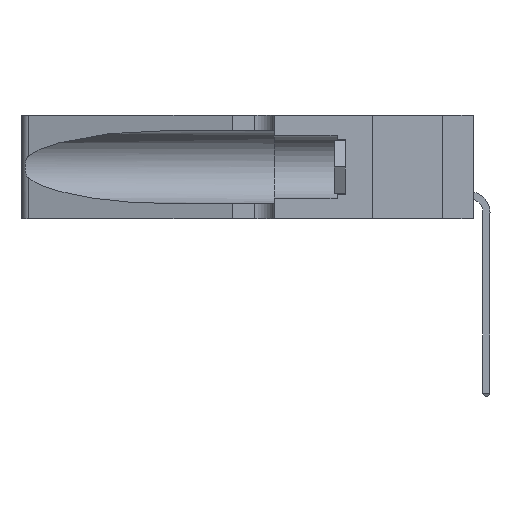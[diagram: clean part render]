
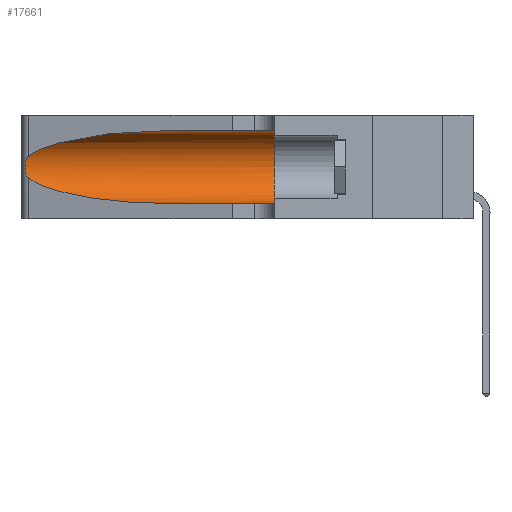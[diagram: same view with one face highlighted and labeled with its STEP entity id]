
A CAD part, left-side view. The second image highlights one B-rep face of the part: STEP entity #17661.
In plain terms, the highlighted cylindrical face has radius 3.308 mm (diameter 6.617 mm), a partial arc.
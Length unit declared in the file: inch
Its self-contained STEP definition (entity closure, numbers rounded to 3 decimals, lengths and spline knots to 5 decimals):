
#1006 = EDGE_CURVE ( 'NONE', #14968, #12927, #1416, .T. ) ;
#1194 = CARTESIAN_POINT ( 'NONE',  ( 0.25487, 1.22718, 0.14631 ) ) ;
#1416 =( BOUNDED_CURVE ( )  B_SPLINE_CURVE ( 3, ( #9014, #8951, #8760, #14597 ),
 .UNSPECIFIED., .F., .F. ) 
 B_SPLINE_CURVE_WITH_KNOTS ( ( 4, 4 ),
 ( 1.5708, 2.84003 ),
 .UNSPECIFIED. ) 
 CURVE ( )  GEOMETRIC_REPRESENTATION_ITEM ( )  RATIONAL_B_SPLINE_CURVE ( ( 1., 0.87, 0.87, 1. ) ) 
 REPRESENTATION_ITEM ( '' )  );
#1436 = EDGE_CURVE ( 'NONE', #14968, #13682, #16048, .T. ) ;
#2096 = CARTESIAN_POINT ( 'NONE',  ( 0.25639, 1.23186, 0.15144 ) ) ;
#2148 = CARTESIAN_POINT ( 'NONE',  ( 0.26017, 1.23833, 0.17102 ) ) ;
#2237 = VERTEX_POINT ( 'NONE', #12793 ) ;
#2344 = EDGE_LOOP ( 'NONE', ( #17675, #3521, #2361, #17129, #5200, #3640 ) ) ;
#2361 = ORIENTED_EDGE ( 'NONE', *, *, #11116, .T. ) ;
#2405 = DIRECTION ( 'NONE',  ( 0., -1., 0. ) ) ;
#2644 = CARTESIAN_POINT ( 'NONE',  ( 0.2373, 1.15595, 0.08982 ) ) ;
#3521 = ORIENTED_EDGE ( 'NONE', *, *, #12593, .T. ) ;
#3640 = ORIENTED_EDGE ( 'NONE', *, *, #1436, .F. ) ;
#4028 = DIRECTION ( 'NONE',  ( 0., 0., 1. ) ) ;
#4147 = DIRECTION ( 'NONE',  ( 0., 1., 0. ) ) ;
#5179 = CARTESIAN_POINT ( 'NONE',  ( 0.1305, 1.61858, 0.185 ) ) ;
#5200 = ORIENTED_EDGE ( 'NONE', *, *, #14529, .F. ) ;
#5296 =( BOUNDED_CURVE ( )  B_SPLINE_CURVE ( 3, ( #1194, #2644, #14162, #15414 ),
 .UNSPECIFIED., .F., .F. ) 
 B_SPLINE_CURVE_WITH_KNOTS ( ( 4, 4 ),
 ( 3.44316, 4.71239 ),
 .UNSPECIFIED. ) 
 CURVE ( )  GEOMETRIC_REPRESENTATION_ITEM ( )  RATIONAL_B_SPLINE_CURVE ( ( 1., 0.87, 0.87, 1. ) ) 
 REPRESENTATION_ITEM ( '' )  );
#6627 = AXIS2_PLACEMENT_3D ( 'NONE', #5179, #2405, #18475 ) ;
#7673 = CARTESIAN_POINT ( 'NONE',  ( 0.25555, 1.22994, 0.2215 ) ) ;
#7732 = CARTESIAN_POINT ( 'NONE',  ( 0.25639, 1.23184, 0.21858 ) ) ;
#7754 = B_SPLINE_CURVE_WITH_KNOTS ( 'NONE', 3,
 ( #16293, #7673, #7732, #17705, #13528, #13592, #17593, #16294, #2148, #8940, #16832, #2096, #17068, #17690 ),
 .UNSPECIFIED., .F., .F.,
 ( 4, 2, 2, 2, 2, 2, 4 ),
 ( 0., 0.00027, 0.00053, 0.00107, 0.0016, 0.00187, 0.00214 ),
 .UNSPECIFIED. ) ;
#8126 = DIRECTION ( 'NONE',  ( 0., -1., 0. ) ) ;
#8757 = EDGE_CURVE ( 'NONE', #2237, #15863, #10971, .T. ) ;
#8760 = CARTESIAN_POINT ( 'NONE',  ( 0.2373, 1.15595, 0.28018 ) ) ;
#8940 = CARTESIAN_POINT ( 'NONE',  ( 0.25856, 1.23593, 0.16098 ) ) ;
#8951 = CARTESIAN_POINT ( 'NONE',  ( 0.18966, 0.96281, 0.31525 ) ) ;
#9014 = CARTESIAN_POINT ( 'NONE',  ( 0.1305, 0.72297, 0.31525 ) ) ;
#9053 = CARTESIAN_POINT ( 'NONE',  ( 0.1305, 0.35, 0.31525 ) ) ;
#9082 = VERTEX_POINT ( 'NONE', #10769 ) ;
#10277 = DIRECTION ( 'NONE',  ( 0., -1., 0. ) ) ;
#10653 = CYLINDRICAL_SURFACE ( 'NONE', #6627, 0.13025 ) ;
#10769 = CARTESIAN_POINT ( 'NONE',  ( 0.25487, 1.22718, 0.14631 ) ) ;
#10971 = LINE ( 'NONE', #13105, #17259 ) ;
#11116 = EDGE_CURVE ( 'NONE', #9082, #2237, #5296, .T. ) ;
#11356 = CIRCLE ( 'NONE', #16221, 0.13025 ) ;
#11788 = FACE_OUTER_BOUND ( 'NONE', #2344, .T. ) ;
#12593 = EDGE_CURVE ( 'NONE', #12927, #9082, #7754, .T. ) ;
#12634 = CARTESIAN_POINT ( 'NONE',  ( 0.1305, 0.72297, 0.31525 ) ) ;
#12793 = CARTESIAN_POINT ( 'NONE',  ( 0.1305, 0.72297, 0.05475 ) ) ;
#12927 = VERTEX_POINT ( 'NONE', #17102 ) ;
#13105 = CARTESIAN_POINT ( 'NONE',  ( 0.1305, 1.61858, 0.05475 ) ) ;
#13528 = CARTESIAN_POINT ( 'NONE',  ( 0.25854, 1.2359, 0.20912 ) ) ;
#13592 = CARTESIAN_POINT ( 'NONE',  ( 0.26018, 1.23835, 0.19895 ) ) ;
#13682 = VERTEX_POINT ( 'NONE', #9053 ) ;
#14162 = CARTESIAN_POINT ( 'NONE',  ( 0.18966, 0.96281, 0.05475 ) ) ;
#14529 = EDGE_CURVE ( 'NONE', #13682, #15863, #11356, .T. ) ;
#14597 = CARTESIAN_POINT ( 'NONE',  ( 0.25487, 1.22718, 0.22369 ) ) ;
#14968 = VERTEX_POINT ( 'NONE', #12634 ) ;
#15414 = CARTESIAN_POINT ( 'NONE',  ( 0.1305, 0.72297, 0.05475 ) ) ;
#15863 = VERTEX_POINT ( 'NONE', #18528 ) ;
#16048 = LINE ( 'NONE', #16290, #18039 ) ;
#16221 = AXIS2_PLACEMENT_3D ( 'NONE', #16879, #4147, #4028 ) ;
#16290 = CARTESIAN_POINT ( 'NONE',  ( 0.1305, 1.61858, 0.31525 ) ) ;
#16293 = CARTESIAN_POINT ( 'NONE',  ( 0.25487, 1.22718, 0.22369 ) ) ;
#16294 = CARTESIAN_POINT ( 'NONE',  ( 0.26075, 1.23896, 0.178 ) ) ;
#16832 = CARTESIAN_POINT ( 'NONE',  ( 0.25789, 1.23486, 0.15765 ) ) ;
#16879 = CARTESIAN_POINT ( 'NONE',  ( 0.1305, 0.35, 0.185 ) ) ;
#17068 = CARTESIAN_POINT ( 'NONE',  ( 0.25555, 1.22993, 0.14849 ) ) ;
#17102 = CARTESIAN_POINT ( 'NONE',  ( 0.25487, 1.22718, 0.22369 ) ) ;
#17129 = ORIENTED_EDGE ( 'NONE', *, *, #8757, .T. ) ;
#17259 = VECTOR ( 'NONE', #10277, 39.37008 ) ;
#17593 = CARTESIAN_POINT ( 'NONE',  ( 0.26075, 1.23896, 0.19203 ) ) ;
#17661 = ADVANCED_FACE ( 'NONE', ( #11788 ), #10653, .F. ) ;
#17675 = ORIENTED_EDGE ( 'NONE', *, *, #1006, .T. ) ;
#17690 = CARTESIAN_POINT ( 'NONE',  ( 0.25487, 1.22718, 0.14631 ) ) ;
#17705 = CARTESIAN_POINT ( 'NONE',  ( 0.25787, 1.23484, 0.2124 ) ) ;
#18039 = VECTOR ( 'NONE', #8126, 39.37008 ) ;
#18475 = DIRECTION ( 'NONE',  ( 0., 0., -1. ) ) ;
#18528 = CARTESIAN_POINT ( 'NONE',  ( 0.1305, 0.35, 0.05475 ) ) ;
